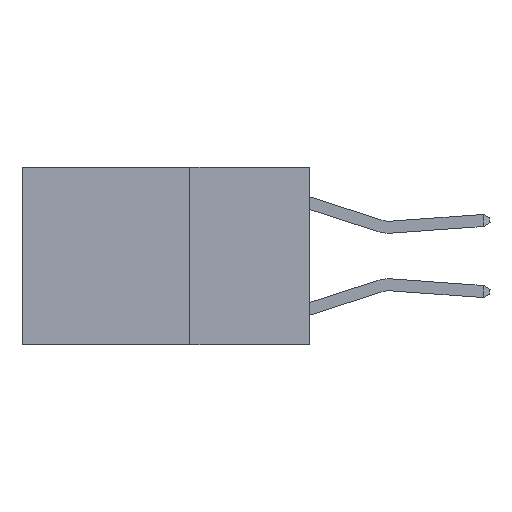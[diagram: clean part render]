
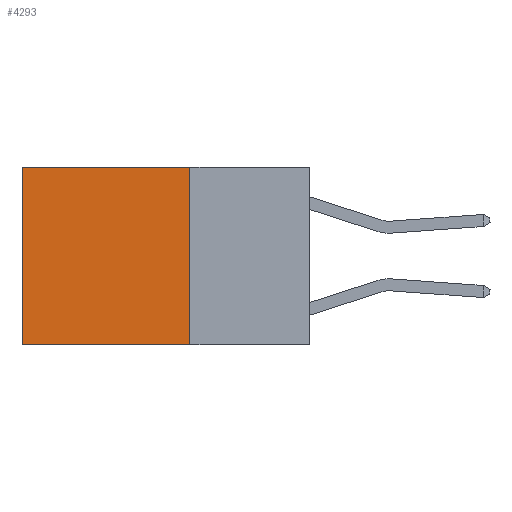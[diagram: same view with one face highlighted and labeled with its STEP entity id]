
A CAD part, left-side view. The second image highlights one B-rep face of the part: STEP entity #4293.
In plain terms, the highlighted planar face has unit normal (-1, 0, 0).
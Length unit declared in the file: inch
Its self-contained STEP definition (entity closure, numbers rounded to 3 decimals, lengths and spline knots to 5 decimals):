
#177 = DIRECTION ( 'NONE',  ( 0., 1., 0. ) ) ;
#435 = VERTEX_POINT ( 'NONE', #8962 ) ;
#946 = EDGE_LOOP ( 'NONE', ( #2620, #1301, #3506, #5683 ) ) ;
#1301 = ORIENTED_EDGE ( 'NONE', *, *, #22825, .F. ) ;
#1313 = EDGE_CURVE ( 'NONE', #18575, #17890, #5188, .T. ) ;
#1483 = CARTESIAN_POINT ( 'NONE',  ( 0.2625, 0.25, -0.37 ) ) ;
#2595 = DIRECTION ( 'NONE',  ( 0., 0., -1. ) ) ;
#2620 = ORIENTED_EDGE ( 'NONE', *, *, #1313, .T. ) ;
#3506 = ORIENTED_EDGE ( 'NONE', *, *, #21087, .F. ) ;
#3658 = CARTESIAN_POINT ( 'NONE',  ( 0.2625, 0.25, 0. ) ) ;
#4293 = ADVANCED_FACE ( 'NONE', ( #8224 ), #15359, .F. ) ;
#4631 = EDGE_CURVE ( 'NONE', #12115, #18575, #16542, .T. ) ;
#5188 = LINE ( 'NONE', #20144, #22867 ) ;
#5683 = ORIENTED_EDGE ( 'NONE', *, *, #4631, .T. ) ;
#8224 = FACE_OUTER_BOUND ( 'NONE', #946, .T. ) ;
#8962 = CARTESIAN_POINT ( 'NONE',  ( 0.2625, 0.25, -0.37 ) ) ;
#9062 = CARTESIAN_POINT ( 'NONE',  ( 0.2625, 0.6, 0. ) ) ;
#10296 = CARTESIAN_POINT ( 'NONE',  ( 0.2625, 0.25, 0. ) ) ;
#10757 = DIRECTION ( 'NONE',  ( 0., 1., 0. ) ) ;
#12115 = VERTEX_POINT ( 'NONE', #23063 ) ;
#12297 = VECTOR ( 'NONE', #10757, 39.37008 ) ;
#13823 = LINE ( 'NONE', #19387, #16816 ) ;
#15359 = PLANE ( 'NONE',  #18675 ) ;
#16306 = VECTOR ( 'NONE', #177, 39.37008 ) ;
#16542 = LINE ( 'NONE', #3658, #16306 ) ;
#16816 = VECTOR ( 'NONE', #19257, 39.37008 ) ;
#16867 = CARTESIAN_POINT ( 'NONE',  ( 0.2625, 0.6, -0.37 ) ) ;
#17663 = DIRECTION ( 'NONE',  ( 1., 0., 0. ) ) ;
#17890 = VERTEX_POINT ( 'NONE', #16867 ) ;
#18575 = VERTEX_POINT ( 'NONE', #9062 ) ;
#18675 = AXIS2_PLACEMENT_3D ( 'NONE', #10296, #17663, #2595 ) ;
#19257 = DIRECTION ( 'NONE',  ( 0., 0., -1. ) ) ;
#19387 = CARTESIAN_POINT ( 'NONE',  ( 0.2625, 0.25, 0. ) ) ;
#19944 = LINE ( 'NONE', #1483, #12297 ) ;
#20144 = CARTESIAN_POINT ( 'NONE',  ( 0.2625, 0.6, 0. ) ) ;
#21087 = EDGE_CURVE ( 'NONE', #12115, #435, #13823, .T. ) ;
#21969 = DIRECTION ( 'NONE',  ( 0., 0., -1. ) ) ;
#22825 = EDGE_CURVE ( 'NONE', #435, #17890, #19944, .T. ) ;
#22867 = VECTOR ( 'NONE', #21969, 39.37008 ) ;
#23063 = CARTESIAN_POINT ( 'NONE',  ( 0.2625, 0.25, 0. ) ) ;
